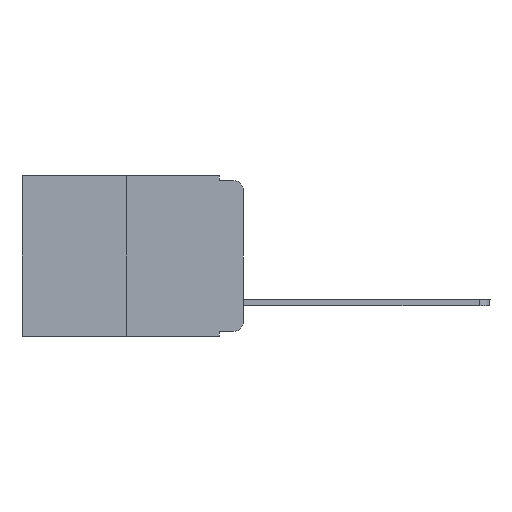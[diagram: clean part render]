
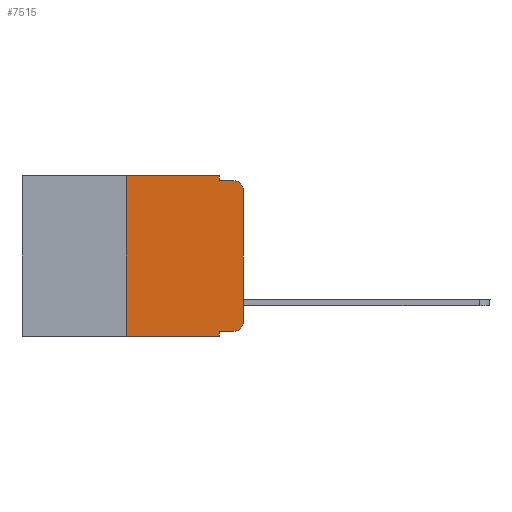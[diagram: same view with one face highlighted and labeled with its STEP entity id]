
A CAD part, left-side view. The second image highlights one B-rep face of the part: STEP entity #7515.
In plain terms, the highlighted planar face has unit normal (-1, 0, 0).
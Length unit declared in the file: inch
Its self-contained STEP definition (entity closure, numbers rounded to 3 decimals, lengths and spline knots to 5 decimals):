
#393 = CIRCLE ( 'NONE', #4588, 0.02 ) ;
#462 = EDGE_CURVE ( 'NONE', #7605, #1443, #6293, .T. ) ;
#595 = ORIENTED_EDGE ( 'NONE', *, *, #6515, .F. ) ;
#905 = ORIENTED_EDGE ( 'NONE', *, *, #10598, .F. ) ;
#1123 = ORIENTED_EDGE ( 'NONE', *, *, #462, .T. ) ;
#1223 = FACE_OUTER_BOUND ( 'NONE', #10275, .T. ) ;
#1342 = VECTOR ( 'NONE', #8354, 39.37008 ) ;
#1404 = VERTEX_POINT ( 'NONE', #8953 ) ;
#1410 = EDGE_CURVE ( 'NONE', #1681, #2665, #5245, .T. ) ;
#1443 = VERTEX_POINT ( 'NONE', #9843 ) ;
#1453 = ORIENTED_EDGE ( 'NONE', *, *, #3197, .F. ) ;
#1458 = ORIENTED_EDGE ( 'NONE', *, *, #10542, .T. ) ;
#1558 = CARTESIAN_POINT ( 'NONE',  ( 0., 0., -0.313 ) ) ;
#1600 = CARTESIAN_POINT ( 'NONE',  ( 0., 0.051, -0.343 ) ) ;
#1681 = VERTEX_POINT ( 'NONE', #6144 ) ;
#1700 = DIRECTION ( 'NONE',  ( 0., 0., -1. ) ) ;
#1769 = CARTESIAN_POINT ( 'NONE',  ( 0., 0.051, -0.01 ) ) ;
#2051 = LINE ( 'NONE', #8291, #10319 ) ;
#2418 = DIRECTION ( 'NONE',  ( 0., -1., 0. ) ) ;
#2665 = VERTEX_POINT ( 'NONE', #9510 ) ;
#2672 = EDGE_CURVE ( 'NONE', #5840, #1404, #4069, .T. ) ;
#2710 = DIRECTION ( 'NONE',  ( 0., 0., -1. ) ) ;
#2957 = LINE ( 'NONE', #4981, #5135 ) ;
#3197 = EDGE_CURVE ( 'NONE', #1404, #7657, #7565, .T. ) ;
#3221 = DIRECTION ( 'NONE',  ( 0., 0., 1. ) ) ;
#3225 = CARTESIAN_POINT ( 'NONE',  ( 0., 0.02, -0.03 ) ) ;
#3231 = CARTESIAN_POINT ( 'NONE',  ( 0., 0.473, 0. ) ) ;
#3348 = LINE ( 'NONE', #1769, #3464 ) ;
#3378 = CARTESIAN_POINT ( 'NONE',  ( 0., 0.051, 0. ) ) ;
#3464 = VECTOR ( 'NONE', #2418, 39.37008 ) ;
#3545 = CARTESIAN_POINT ( 'NONE',  ( 0., 0.02, -0.313 ) ) ;
#3778 = CIRCLE ( 'NONE', #4168, 0.02 ) ;
#3994 = CARTESIAN_POINT ( 'NONE',  ( 0., 0.051, -0.333 ) ) ;
#4069 = LINE ( 'NONE', #4572, #5473 ) ;
#4168 = AXIS2_PLACEMENT_3D ( 'NONE', #3225, #4179, #6546 ) ;
#4177 = EDGE_CURVE ( 'NONE', #1443, #8503, #3778, .T. ) ;
#4179 = DIRECTION ( 'NONE',  ( -1., 0., 0. ) ) ;
#4183 = CARTESIAN_POINT ( 'NONE',  ( 0., 0.25, 0. ) ) ;
#4362 = VECTOR ( 'NONE', #3221, 39.37008 ) ;
#4424 = DIRECTION ( 'NONE',  ( -1., 0., 0. ) ) ;
#4572 = CARTESIAN_POINT ( 'NONE',  ( 0., 0.473, 0. ) ) ;
#4588 = AXIS2_PLACEMENT_3D ( 'NONE', #3545, #4424, #2710 ) ;
#4825 = VERTEX_POINT ( 'NONE', #1600 ) ;
#4972 = ORIENTED_EDGE ( 'NONE', *, *, #1410, .T. ) ;
#4975 = VECTOR ( 'NONE', #10627, 39.37008 ) ;
#4978 = EDGE_CURVE ( 'NONE', #7657, #8503, #3348, .T. ) ;
#4981 = CARTESIAN_POINT ( 'NONE',  ( 0., 0.473, -0.343 ) ) ;
#5135 = VECTOR ( 'NONE', #6539, 39.37008 ) ;
#5245 = LINE ( 'NONE', #3994, #4975 ) ;
#5434 = CARTESIAN_POINT ( 'NONE',  ( 0., 0.25, -0.343 ) ) ;
#5473 = VECTOR ( 'NONE', #9474, 39.37008 ) ;
#5649 = CARTESIAN_POINT ( 'NONE',  ( 0., 0.02, -0.01 ) ) ;
#5712 = DIRECTION ( 'NONE',  ( 0., 0., -1. ) ) ;
#5713 = CARTESIAN_POINT ( 'NONE',  ( 0., 0., 0. ) ) ;
#5840 = VERTEX_POINT ( 'NONE', #4183 ) ;
#6144 = CARTESIAN_POINT ( 'NONE',  ( 0., 0.051, -0.333 ) ) ;
#6293 = LINE ( 'NONE', #5713, #4362 ) ;
#6406 = ORIENTED_EDGE ( 'NONE', *, *, #4177, .T. ) ;
#6515 = EDGE_CURVE ( 'NONE', #10379, #5840, #9523, .T. ) ;
#6539 = DIRECTION ( 'NONE',  ( 0., -1., 0. ) ) ;
#6546 = DIRECTION ( 'NONE',  ( 0., 0., -1. ) ) ;
#6926 = CARTESIAN_POINT ( 'NONE',  ( 0., 0.25, 0. ) ) ;
#6927 = AXIS2_PLACEMENT_3D ( 'NONE', #3231, #9934, #1700 ) ;
#7515 = ADVANCED_FACE ( 'NONE', ( #1223 ), #9137, .F. ) ;
#7565 = LINE ( 'NONE', #3378, #1342 ) ;
#7605 = VERTEX_POINT ( 'NONE', #1558 ) ;
#7657 = VERTEX_POINT ( 'NONE', #10030 ) ;
#7846 = ORIENTED_EDGE ( 'NONE', *, *, #9526, .T. ) ;
#8291 = CARTESIAN_POINT ( 'NONE',  ( 0., 0.051, 0. ) ) ;
#8354 = DIRECTION ( 'NONE',  ( 0., 0., -1. ) ) ;
#8503 = VERTEX_POINT ( 'NONE', #5649 ) ;
#8700 = ORIENTED_EDGE ( 'NONE', *, *, #4978, .F. ) ;
#8953 = CARTESIAN_POINT ( 'NONE',  ( 0., 0.051, 0. ) ) ;
#9137 = PLANE ( 'NONE',  #6927 ) ;
#9474 = DIRECTION ( 'NONE',  ( 0., -1., 0. ) ) ;
#9510 = CARTESIAN_POINT ( 'NONE',  ( 0., 0.02, -0.333 ) ) ;
#9523 = LINE ( 'NONE', #6926, #10277 ) ;
#9526 = EDGE_CURVE ( 'NONE', #2665, #7605, #393, .T. ) ;
#9723 = ORIENTED_EDGE ( 'NONE', *, *, #2672, .F. ) ;
#9843 = CARTESIAN_POINT ( 'NONE',  ( 0., 0., -0.03 ) ) ;
#9934 = DIRECTION ( 'NONE',  ( 1., 0., 0. ) ) ;
#10030 = CARTESIAN_POINT ( 'NONE',  ( 0., 0.051, -0.01 ) ) ;
#10152 = DIRECTION ( 'NONE',  ( 0., 0., 1. ) ) ;
#10275 = EDGE_LOOP ( 'NONE', ( #1123, #6406, #8700, #1453, #9723, #595, #1458, #905, #4972, #7846 ) ) ;
#10277 = VECTOR ( 'NONE', #10152, 39.37008 ) ;
#10319 = VECTOR ( 'NONE', #5712, 39.37008 ) ;
#10379 = VERTEX_POINT ( 'NONE', #5434 ) ;
#10542 = EDGE_CURVE ( 'NONE', #10379, #4825, #2957, .T. ) ;
#10598 = EDGE_CURVE ( 'NONE', #1681, #4825, #2051, .T. ) ;
#10627 = DIRECTION ( 'NONE',  ( 0., -1., 0. ) ) ;
